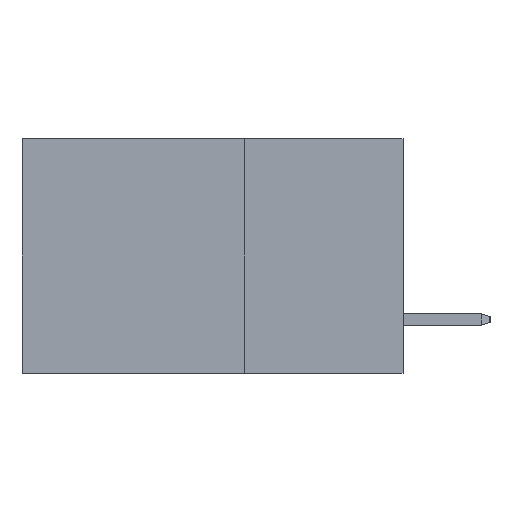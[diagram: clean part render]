
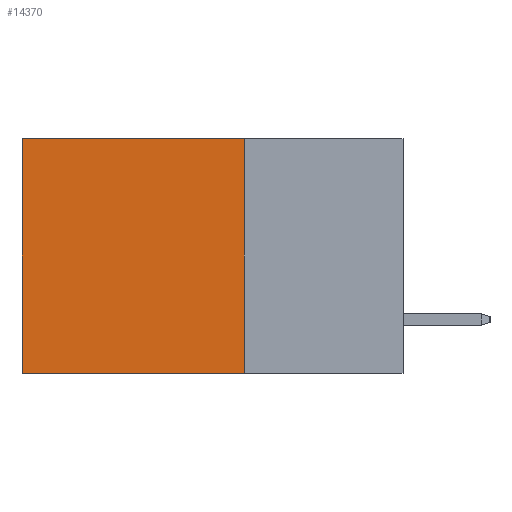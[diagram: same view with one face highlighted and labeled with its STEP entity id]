
A CAD part, left-side view. The second image highlights one B-rep face of the part: STEP entity #14370.
In plain terms, the highlighted planar face has unit normal (-1, 0, 0).
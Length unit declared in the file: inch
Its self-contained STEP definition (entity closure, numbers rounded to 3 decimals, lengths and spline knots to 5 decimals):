
#6 = CARTESIAN_POINT ( 'NONE',  ( 0.2875, 0.6, 0. ) ) ;
#773 = AXIS2_PLACEMENT_3D ( 'NONE', #8282, #4745, #9150 ) ;
#962 = CARTESIAN_POINT ( 'NONE',  ( 0.2875, 0.25, -0.37 ) ) ;
#984 = ORIENTED_EDGE ( 'NONE', *, *, #13212, .T. ) ;
#1295 = CARTESIAN_POINT ( 'NONE',  ( 0.2875, 0.25, 0. ) ) ;
#2779 = VECTOR ( 'NONE', #11251, 39.37008 ) ;
#3794 = LINE ( 'NONE', #5094, #13021 ) ;
#4423 = LINE ( 'NONE', #6, #14198 ) ;
#4745 = DIRECTION ( 'NONE',  ( 1., 0., 0. ) ) ;
#5094 = CARTESIAN_POINT ( 'NONE',  ( 0.2875, 0.25, 0. ) ) ;
#6709 = VERTEX_POINT ( 'NONE', #6894 ) ;
#6715 = VECTOR ( 'NONE', #11210, 39.37008 ) ;
#6894 = CARTESIAN_POINT ( 'NONE',  ( 0.2875, 0.6, 0. ) ) ;
#6980 = DIRECTION ( 'NONE',  ( 0., 1., 0. ) ) ;
#7064 = FACE_OUTER_BOUND ( 'NONE', #12913, .T. ) ;
#7559 = EDGE_CURVE ( 'NONE', #12749, #12671, #7792, .T. ) ;
#7792 = LINE ( 'NONE', #13186, #6715 ) ;
#8137 = ORIENTED_EDGE ( 'NONE', *, *, #7559, .F. ) ;
#8282 = CARTESIAN_POINT ( 'NONE',  ( 0.2875, 0.25, 0. ) ) ;
#9150 = DIRECTION ( 'NONE',  ( 0., 0., -1. ) ) ;
#11178 = EDGE_CURVE ( 'NONE', #12942, #12749, #11326, .T. ) ;
#11210 = DIRECTION ( 'NONE',  ( 0., 1., 0. ) ) ;
#11251 = DIRECTION ( 'NONE',  ( 0., 0., -1. ) ) ;
#11257 = EDGE_CURVE ( 'NONE', #12942, #6709, #3794, .T. ) ;
#11326 = LINE ( 'NONE', #13369, #2779 ) ;
#11507 = ORIENTED_EDGE ( 'NONE', *, *, #11178, .F. ) ;
#12270 = DIRECTION ( 'NONE',  ( 0., 0., -1. ) ) ;
#12523 = PLANE ( 'NONE',  #773 ) ;
#12671 = VERTEX_POINT ( 'NONE', #13032 ) ;
#12749 = VERTEX_POINT ( 'NONE', #962 ) ;
#12913 = EDGE_LOOP ( 'NONE', ( #984, #8137, #11507, #13207 ) ) ;
#12942 = VERTEX_POINT ( 'NONE', #1295 ) ;
#13021 = VECTOR ( 'NONE', #6980, 39.37008 ) ;
#13032 = CARTESIAN_POINT ( 'NONE',  ( 0.2875, 0.6, -0.37 ) ) ;
#13186 = CARTESIAN_POINT ( 'NONE',  ( 0.2875, 0.25, -0.37 ) ) ;
#13207 = ORIENTED_EDGE ( 'NONE', *, *, #11257, .T. ) ;
#13212 = EDGE_CURVE ( 'NONE', #6709, #12671, #4423, .T. ) ;
#13369 = CARTESIAN_POINT ( 'NONE',  ( 0.2875, 0.25, 0. ) ) ;
#14198 = VECTOR ( 'NONE', #12270, 39.37008 ) ;
#14370 = ADVANCED_FACE ( 'NONE', ( #7064 ), #12523, .F. ) ;
